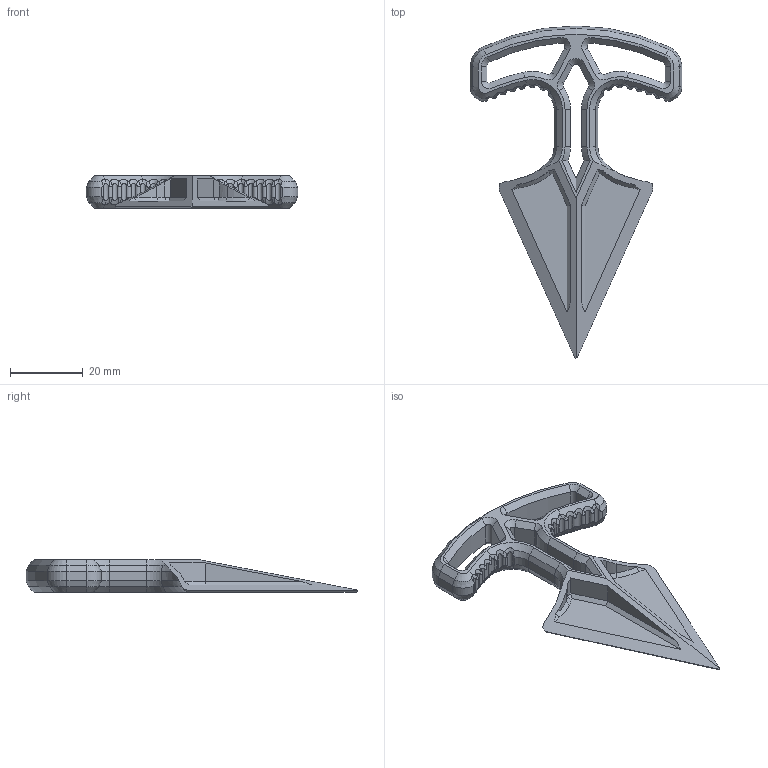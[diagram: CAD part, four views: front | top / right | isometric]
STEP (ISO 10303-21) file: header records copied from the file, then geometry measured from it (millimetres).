
FILE_DESCRIPTION(/* description */ (''),/* implementation_level */ '2;1');
FILE_NAME(/* name */ 'Malice.step',/* time_stamp */ '2021-09-20T13:39:20-04:00',/* author */ (''),/* organization */ (''),/* preprocessor_version */ 'ST-DEVELOPER v18.1',/* originating_system */ 'Autodesk Translation Framework v10.10.0.1391',/* authorisation */ '');
FILE_SCHEMA (('AUTOMOTIVE_DESIGN { 1 0 10303 214 3 1 1 }'));
Length unit declared in the file: millimetre
Products named in the file (1): Malice
Bounding box: 58 x 91.01 x 9 mm (x, y, z)
Volume: 8925.3 mm3; surface area: 6822.9 mm2
Topology: 1 solids, 1 shells, 308 faces, 786 edges, 482 vertices
Faces by surface type: cone 118, cylinder 76, plane 73, bspline 41
Entity records: 14814 total; most frequent: CARTESIAN_POINT 7818, ORIENTED_EDGE 1572, DIRECTION 1279, EDGE_CURVE 786, VERTEX_POINT 482, AXIS2_PLACEMENT_3D 480, LINE 319, VECTOR 319
